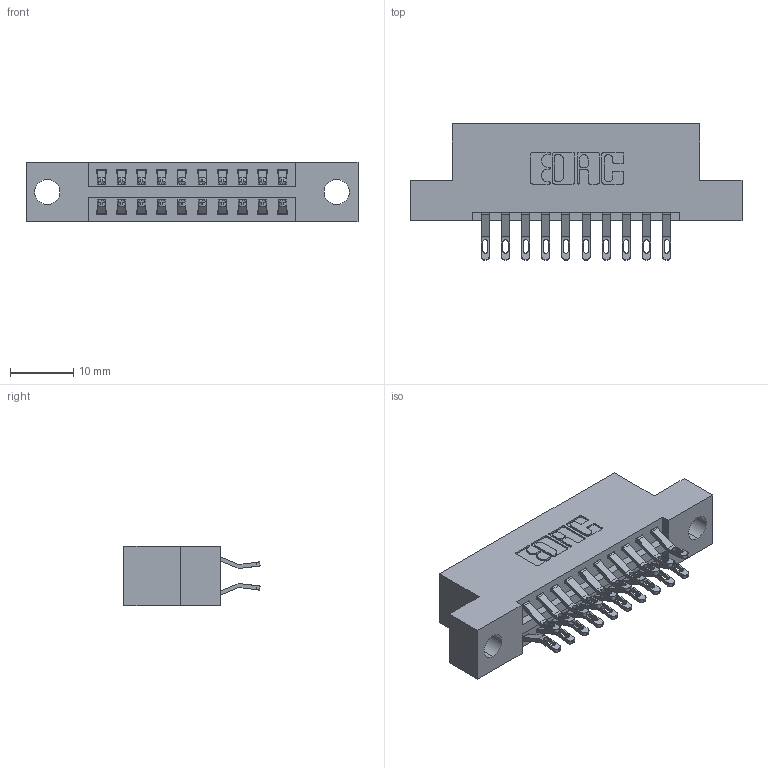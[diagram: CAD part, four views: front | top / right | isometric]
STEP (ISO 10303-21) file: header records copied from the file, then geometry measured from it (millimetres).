
FILE_DESCRIPTION (( 'STEP AP203' ), '1' );
FILE_NAME ('396-020-555-204.STEP', '2018-09-01T06:18:13', ( '' ), ( '' ), 'SwSTEP 2.0', 'SolidWorks 2016', '' );
FILE_SCHEMA (( 'CONFIG_CONTROL_DESIGN' ));
Length unit declared in the file: inch
Products named in the file (3): 346 Part_Flush Mounting Lugs - 0.156 Dia-TH; 345-292-001_555 Tail; 396-020-555-204
Assembly tree (21 placements, depth 2):
  396-020-555-204
    346 Part_Flush Mounting Lugs - 0.156 Dia-TH
    345-292-001_555 Tail  x20
Bounding box: 52.32 x 21.46 x 9.4 mm (x, y, z)
Volume: 4823.9 mm3; surface area: 6147.9 mm2
Topology: 21 solids, 21 shells, 1282 faces, 3989 edges, 2658 vertices
Faces by surface type: plane 736, cylinder 546
Entity records: 11163 total; most frequent: CARTESIAN_POINT 1918, ORIENTED_EDGE 1822, DIRECTION 1711, EDGE_CURVE 911, LINE 719, VECTOR 719, VERTEX_POINT 606, AXIS2_PLACEMENT_3D 496
